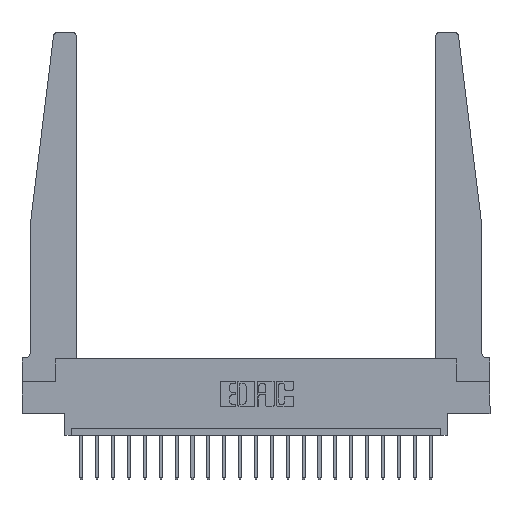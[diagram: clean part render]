
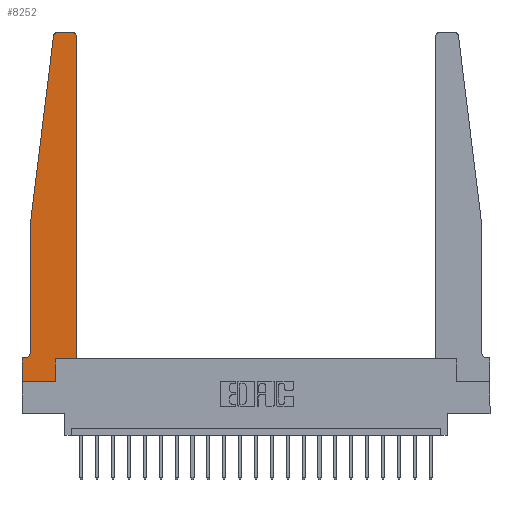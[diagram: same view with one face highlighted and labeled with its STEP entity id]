
A CAD part, top view. The second image highlights one B-rep face of the part: STEP entity #8252.
In plain terms, the highlighted planar face has unit normal (0, 0, 1).
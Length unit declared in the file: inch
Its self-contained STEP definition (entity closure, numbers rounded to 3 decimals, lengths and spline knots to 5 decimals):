
#32 = VERTEX_POINT ( 'NONE', #11287 ) ;
#187 = VECTOR ( 'NONE', #19647, 39.37008 ) ;
#279 = DIRECTION ( 'NONE',  ( -0.122, -0.992, 0. ) ) ;
#358 = EDGE_CURVE ( 'NONE', #8679, #32, #12270, .T. ) ;
#444 = CARTESIAN_POINT ( 'NONE',  ( 0.425, 0.18, 0.37 ) ) ;
#676 = CARTESIAN_POINT ( 'NONE',  ( 0.27653, 2.75, 0.37 ) ) ;
#1893 = CARTESIAN_POINT ( 'NONE',  ( 0.425, 0.18, 0.37 ) ) ;
#1990 = LINE ( 'NONE', #19228, #9982 ) ;
#2117 = VECTOR ( 'NONE', #12428, 39.37008 ) ;
#2313 = VERTEX_POINT ( 'NONE', #4727 ) ;
#2430 = EDGE_CURVE ( 'NONE', #15941, #2313, #17009, .T. ) ;
#2644 = DIRECTION ( 'NONE',  ( 0., 1., 0. ) ) ;
#2870 = CARTESIAN_POINT ( 'NONE',  ( 0.425, 2.72, 0.37 ) ) ;
#2949 = VERTEX_POINT ( 'NONE', #14068 ) ;
#3131 = CARTESIAN_POINT ( 'NONE',  ( 0.065, 0.1875, 0.37 ) ) ;
#3180 = CARTESIAN_POINT ( 'NONE',  ( 0.27653, 2.72, 0.37 ) ) ;
#3516 = DIRECTION ( 'NONE',  ( 1., 0., 0. ) ) ;
#3529 = DIRECTION ( 'NONE',  ( 0., 0., 1. ) ) ;
#3884 = CARTESIAN_POINT ( 'NONE',  ( 0., 0., 0.37 ) ) ;
#3902 = DIRECTION ( 'NONE',  ( 0., 0., -1. ) ) ;
#3966 = PLANE ( 'NONE',  #11628 ) ;
#4215 = CARTESIAN_POINT ( 'NONE',  ( 0.2605, 0.18, 0.37 ) ) ;
#4264 = EDGE_CURVE ( 'NONE', #19756, #16801, #7479, .T. ) ;
#4544 = LINE ( 'NONE', #19757, #187 ) ;
#4727 = CARTESIAN_POINT ( 'NONE',  ( 0.425, 0.18, 0.37 ) ) ;
#5054 = VERTEX_POINT ( 'NONE', #21422 ) ;
#5483 = ORIENTED_EDGE ( 'NONE', *, *, #2430, .T. ) ;
#5677 = DIRECTION ( 'NONE',  ( 0., -1., 0. ) ) ;
#5752 = CARTESIAN_POINT ( 'NONE',  ( 0.395, 2.75, 0.37 ) ) ;
#5883 = VERTEX_POINT ( 'NONE', #18004 ) ;
#6061 = VERTEX_POINT ( 'NONE', #9044 ) ;
#6233 = EDGE_CURVE ( 'NONE', #5054, #2949, #13825, .T. ) ;
#6606 = LINE ( 'NONE', #3131, #17568 ) ;
#7284 = EDGE_CURVE ( 'NONE', #2949, #5883, #6606, .T. ) ;
#7479 = LINE ( 'NONE', #14071, #15055 ) ;
#7800 = LINE ( 'NONE', #3884, #9622 ) ;
#7941 = EDGE_CURVE ( 'NONE', #32, #5054, #4544, .T. ) ;
#8252 = ADVANCED_FACE ( 'NONE', ( #12449 ), #3966, .T. ) ;
#8433 = VECTOR ( 'NONE', #279, 39.37008 ) ;
#8679 = VERTEX_POINT ( 'NONE', #15963 ) ;
#8837 = ORIENTED_EDGE ( 'NONE', *, *, #14474, .T. ) ;
#8849 = ORIENTED_EDGE ( 'NONE', *, *, #11838, .T. ) ;
#9044 = CARTESIAN_POINT ( 'NONE',  ( 0.2605, 0., 0.37 ) ) ;
#9173 = VECTOR ( 'NONE', #10128, 39.37008 ) ;
#9238 = VERTEX_POINT ( 'NONE', #2870 ) ;
#9468 = ORIENTED_EDGE ( 'NONE', *, *, #19423, .T. ) ;
#9622 = VECTOR ( 'NONE', #21238, 39.37008 ) ;
#9756 = EDGE_CURVE ( 'NONE', #16801, #8679, #12046, .T. ) ;
#9982 = VECTOR ( 'NONE', #5677, 39.37008 ) ;
#10128 = DIRECTION ( 'NONE',  ( 1., 0., 0. ) ) ;
#10389 = DIRECTION ( 'NONE',  ( -1., 0., 0. ) ) ;
#10775 = DIRECTION ( 'NONE',  ( 1., 0., 0. ) ) ;
#10806 = ORIENTED_EDGE ( 'NONE', *, *, #358, .T. ) ;
#11287 = CARTESIAN_POINT ( 'NONE',  ( 0.065, 1.25, 0.37 ) ) ;
#11407 = DIRECTION ( 'NONE',  ( 1., 0., 0. ) ) ;
#11628 = AXIS2_PLACEMENT_3D ( 'NONE', #17387, #3529, #10775 ) ;
#11838 = EDGE_CURVE ( 'NONE', #9238, #19756, #18530, .T. ) ;
#12042 = EDGE_CURVE ( 'NONE', #5883, #19383, #1990, .T. ) ;
#12046 = CIRCLE ( 'NONE', #12386, 0.03 ) ;
#12270 = LINE ( 'NONE', #20916, #8433 ) ;
#12386 = AXIS2_PLACEMENT_3D ( 'NONE', #3180, #20422, #3516 ) ;
#12428 = DIRECTION ( 'NONE',  ( 0., 1., 0. ) ) ;
#12449 = FACE_OUTER_BOUND ( 'NONE', #14325, .T. ) ;
#12751 = AXIS2_PLACEMENT_3D ( 'NONE', #15957, #3902, #10389 ) ;
#13490 = ORIENTED_EDGE ( 'NONE', *, *, #6233, .T. ) ;
#13693 = EDGE_CURVE ( 'NONE', #19383, #6061, #7800, .T. ) ;
#13825 = CIRCLE ( 'NONE', #12751, 0.05 ) ;
#14068 = CARTESIAN_POINT ( 'NONE',  ( 0.015, 0.1875, 0.37 ) ) ;
#14071 = CARTESIAN_POINT ( 'NONE',  ( 0.25, 2.75, 0.37 ) ) ;
#14325 = EDGE_LOOP ( 'NONE', ( #14484, #17399, #10806, #18298, #13490, #14885, #21159, #20653, #9468, #5483, #8837, #8849 ) ) ;
#14474 = EDGE_CURVE ( 'NONE', #2313, #9238, #16119, .T. ) ;
#14484 = ORIENTED_EDGE ( 'NONE', *, *, #4264, .T. ) ;
#14615 = LINE ( 'NONE', #4215, #19451 ) ;
#14885 = ORIENTED_EDGE ( 'NONE', *, *, #7284, .T. ) ;
#15055 = VECTOR ( 'NONE', #20925, 39.37008 ) ;
#15091 = DIRECTION ( 'NONE',  ( -1., 0., 0. ) ) ;
#15941 = VERTEX_POINT ( 'NONE', #20279 ) ;
#15957 = CARTESIAN_POINT ( 'NONE',  ( 0.015, 0.2375, 0.37 ) ) ;
#15963 = CARTESIAN_POINT ( 'NONE',  ( 0.24675, 2.72367, 0.37 ) ) ;
#16119 = LINE ( 'NONE', #444, #2117 ) ;
#16284 = CARTESIAN_POINT ( 'NONE',  ( 0., 0., 0.37 ) ) ;
#16801 = VERTEX_POINT ( 'NONE', #676 ) ;
#17009 = LINE ( 'NONE', #1893, #9173 ) ;
#17387 = CARTESIAN_POINT ( 'NONE',  ( 0., 0.1875, 0.37 ) ) ;
#17399 = ORIENTED_EDGE ( 'NONE', *, *, #9756, .T. ) ;
#17568 = VECTOR ( 'NONE', #15091, 39.37008 ) ;
#18001 = CARTESIAN_POINT ( 'NONE',  ( 0.395, 2.72, 0.37 ) ) ;
#18004 = CARTESIAN_POINT ( 'NONE',  ( 0., 0.1875, 0.37 ) ) ;
#18110 = DIRECTION ( 'NONE',  ( 0., 0., 1. ) ) ;
#18169 = AXIS2_PLACEMENT_3D ( 'NONE', #18001, #18110, #11407 ) ;
#18298 = ORIENTED_EDGE ( 'NONE', *, *, #7941, .T. ) ;
#18530 = CIRCLE ( 'NONE', #18169, 0.03 ) ;
#19228 = CARTESIAN_POINT ( 'NONE',  ( 0., 0., 0.37 ) ) ;
#19383 = VERTEX_POINT ( 'NONE', #16284 ) ;
#19423 = EDGE_CURVE ( 'NONE', #6061, #15941, #14615, .T. ) ;
#19451 = VECTOR ( 'NONE', #2644, 39.37008 ) ;
#19647 = DIRECTION ( 'NONE',  ( 0., -1., 0. ) ) ;
#19756 = VERTEX_POINT ( 'NONE', #5752 ) ;
#19757 = CARTESIAN_POINT ( 'NONE',  ( 0.065, 1.25, 0.37 ) ) ;
#20279 = CARTESIAN_POINT ( 'NONE',  ( 0.2605, 0.18, 0.37 ) ) ;
#20422 = DIRECTION ( 'NONE',  ( 0., 0., 1. ) ) ;
#20653 = ORIENTED_EDGE ( 'NONE', *, *, #13693, .T. ) ;
#20916 = CARTESIAN_POINT ( 'NONE',  ( 0.065, 1.25, 0.37 ) ) ;
#20925 = DIRECTION ( 'NONE',  ( -1., 0., 0. ) ) ;
#21159 = ORIENTED_EDGE ( 'NONE', *, *, #12042, .T. ) ;
#21238 = DIRECTION ( 'NONE',  ( 1., 0., 0. ) ) ;
#21422 = CARTESIAN_POINT ( 'NONE',  ( 0.065, 0.2375, 0.37 ) ) ;
